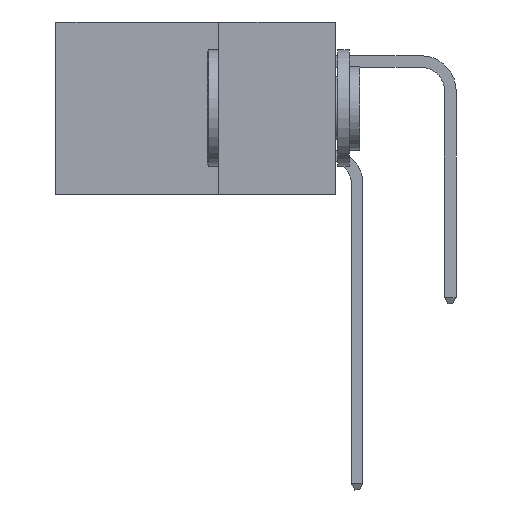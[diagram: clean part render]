
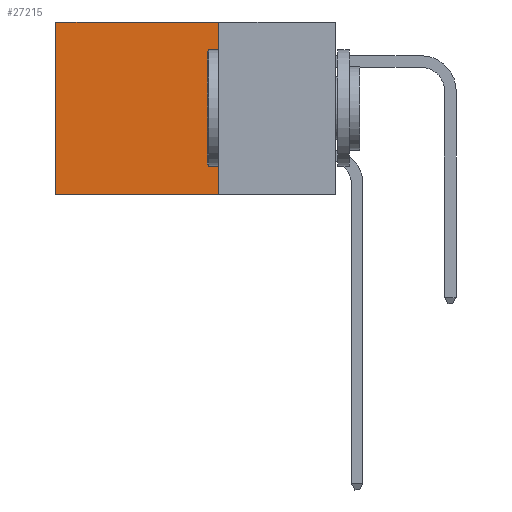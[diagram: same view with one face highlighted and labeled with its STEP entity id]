
A CAD part, left-side view. The second image highlights one B-rep face of the part: STEP entity #27215.
In plain terms, the highlighted planar face has unit normal (-1, 0, 0).
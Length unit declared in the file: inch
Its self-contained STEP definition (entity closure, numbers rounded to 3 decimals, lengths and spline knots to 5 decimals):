
#230 = CARTESIAN_POINT ( 'NONE',  ( 0.2875, 0.6, -0.37 ) ) ;
#463 = DIRECTION ( 'NONE',  ( 0., 0., -1. ) ) ;
#1873 = EDGE_CURVE ( 'NONE', #6403, #5553, #33423, .T. ) ;
#2036 = AXIS2_PLACEMENT_3D ( 'NONE', #30212, #6198, #12451 ) ;
#3025 = LINE ( 'NONE', #16559, #9985 ) ;
#3317 = EDGE_CURVE ( 'NONE', #18415, #5553, #3025, .T. ) ;
#5553 = VERTEX_POINT ( 'NONE', #230 ) ;
#6065 = VECTOR ( 'NONE', #31874, 39.37008 ) ;
#6198 = DIRECTION ( 'NONE',  ( 1., 0., 0. ) ) ;
#6403 = VERTEX_POINT ( 'NONE', #34319 ) ;
#6416 = ORIENTED_EDGE ( 'NONE', *, *, #7344, .T. ) ;
#7344 = EDGE_CURVE ( 'NONE', #29851, #6403, #11098, .T. ) ;
#8084 = CARTESIAN_POINT ( 'NONE',  ( 0.2875, 0.25, 0. ) ) ;
#9985 = VECTOR ( 'NONE', #25523, 39.37008 ) ;
#11098 = LINE ( 'NONE', #14254, #19727 ) ;
#12451 = DIRECTION ( 'NONE',  ( 0., 0., -1. ) ) ;
#14254 = CARTESIAN_POINT ( 'NONE',  ( 0.2875, 0.25, 0. ) ) ;
#14439 = CARTESIAN_POINT ( 'NONE',  ( 0.2875, 0.25, -0.37 ) ) ;
#15955 = CARTESIAN_POINT ( 'NONE',  ( 0.2875, 0.25, 0. ) ) ;
#16559 = CARTESIAN_POINT ( 'NONE',  ( 0.2875, 0.25, -0.37 ) ) ;
#18415 = VERTEX_POINT ( 'NONE', #14439 ) ;
#19205 = ORIENTED_EDGE ( 'NONE', *, *, #30764, .F. ) ;
#19727 = VECTOR ( 'NONE', #37673, 39.37008 ) ;
#20471 = ORIENTED_EDGE ( 'NONE', *, *, #3317, .F. ) ;
#24265 = CARTESIAN_POINT ( 'NONE',  ( 0.2875, 0.6, 0. ) ) ;
#25505 = VECTOR ( 'NONE', #463, 39.37008 ) ;
#25523 = DIRECTION ( 'NONE',  ( 0., 1., 0. ) ) ;
#27215 = ADVANCED_FACE ( 'NONE', ( #30188 ), #27247, .F. ) ;
#27247 = PLANE ( 'NONE',  #2036 ) ;
#29619 = EDGE_LOOP ( 'NONE', ( #34050, #20471, #19205, #6416 ) ) ;
#29851 = VERTEX_POINT ( 'NONE', #15955 ) ;
#30188 = FACE_OUTER_BOUND ( 'NONE', #29619, .T. ) ;
#30212 = CARTESIAN_POINT ( 'NONE',  ( 0.2875, 0.25, 0. ) ) ;
#30764 = EDGE_CURVE ( 'NONE', #29851, #18415, #33510, .T. ) ;
#31874 = DIRECTION ( 'NONE',  ( 0., 0., -1. ) ) ;
#33423 = LINE ( 'NONE', #24265, #25505 ) ;
#33510 = LINE ( 'NONE', #8084, #6065 ) ;
#34050 = ORIENTED_EDGE ( 'NONE', *, *, #1873, .T. ) ;
#34319 = CARTESIAN_POINT ( 'NONE',  ( 0.2875, 0.6, 0. ) ) ;
#37673 = DIRECTION ( 'NONE',  ( 0., 1., 0. ) ) ;
